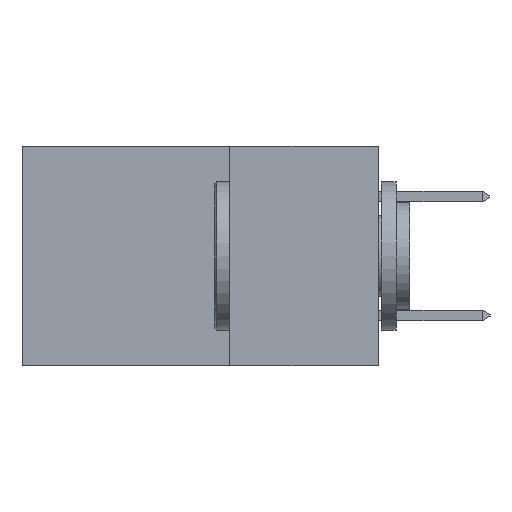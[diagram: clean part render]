
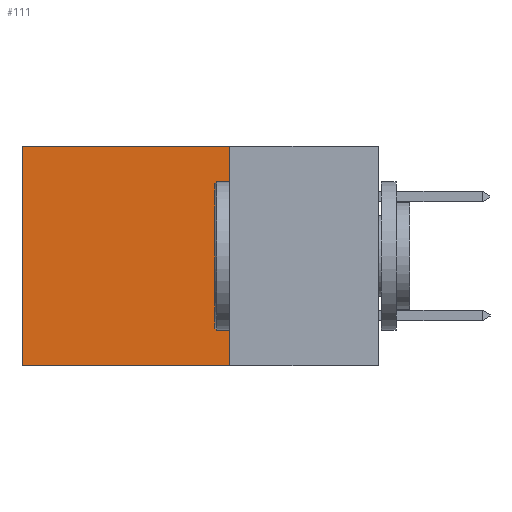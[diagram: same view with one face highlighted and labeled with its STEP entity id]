
A CAD part, left-side view. The second image highlights one B-rep face of the part: STEP entity #111.
In plain terms, the highlighted planar face has unit normal (-1, 0, 0).
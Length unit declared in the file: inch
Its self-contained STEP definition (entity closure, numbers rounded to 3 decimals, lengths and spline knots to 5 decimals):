
#111 = ADVANCED_FACE ( 'NONE', ( #12566 ), #7106, .F. ) ;
#1089 = CARTESIAN_POINT ( 'NONE',  ( 0.2615, 0.25, -0.37 ) ) ;
#1488 = EDGE_CURVE ( 'NONE', #8205, #7465, #5179, .T. ) ;
#1887 = VECTOR ( 'NONE', #9534, 39.37008 ) ;
#2770 = LINE ( 'NONE', #9122, #12770 ) ;
#3775 = CARTESIAN_POINT ( 'NONE',  ( 0.2615, 0.25, -0.37 ) ) ;
#3989 = DIRECTION ( 'NONE',  ( 0., 0., -1. ) ) ;
#4307 = EDGE_LOOP ( 'NONE', ( #10764, #14239, #8349, #5482 ) ) ;
#4802 = VERTEX_POINT ( 'NONE', #9299 ) ;
#4962 = CARTESIAN_POINT ( 'NONE',  ( 0.2615, 0.25, -0.37 ) ) ;
#5179 = LINE ( 'NONE', #13871, #1887 ) ;
#5255 = LINE ( 'NONE', #3775, #11682 ) ;
#5482 = ORIENTED_EDGE ( 'NONE', *, *, #6745, .T. ) ;
#6457 = DIRECTION ( 'NONE',  ( 0., 0., -1. ) ) ;
#6491 = DIRECTION ( 'NONE',  ( 1., 0., 0. ) ) ;
#6745 = EDGE_CURVE ( 'NONE', #4802, #8205, #14173, .T. ) ;
#7106 = PLANE ( 'NONE',  #14332 ) ;
#7465 = VERTEX_POINT ( 'NONE', #13145 ) ;
#7896 = VECTOR ( 'NONE', #8722, 39.37008 ) ;
#8205 = VERTEX_POINT ( 'NONE', #10181 ) ;
#8349 = ORIENTED_EDGE ( 'NONE', *, *, #10318, .F. ) ;
#8722 = DIRECTION ( 'NONE',  ( 0., 1., 0. ) ) ;
#8735 = DIRECTION ( 'NONE',  ( 0., 1., 0. ) ) ;
#9122 = CARTESIAN_POINT ( 'NONE',  ( 0.2615, 0.25, -0.37 ) ) ;
#9299 = CARTESIAN_POINT ( 'NONE',  ( 0.2615, 0.25, 0. ) ) ;
#9534 = DIRECTION ( 'NONE',  ( 0., 0., -1. ) ) ;
#10181 = CARTESIAN_POINT ( 'NONE',  ( 0.2615, 0.6, 0. ) ) ;
#10318 = EDGE_CURVE ( 'NONE', #4802, #11355, #5255, .T. ) ;
#10723 = EDGE_CURVE ( 'NONE', #11355, #7465, #2770, .T. ) ;
#10764 = ORIENTED_EDGE ( 'NONE', *, *, #1488, .T. ) ;
#11340 = CARTESIAN_POINT ( 'NONE',  ( 0.2615, 0.25, 0. ) ) ;
#11355 = VERTEX_POINT ( 'NONE', #1089 ) ;
#11682 = VECTOR ( 'NONE', #3989, 39.37008 ) ;
#12566 = FACE_OUTER_BOUND ( 'NONE', #4307, .T. ) ;
#12770 = VECTOR ( 'NONE', #8735, 39.37008 ) ;
#13145 = CARTESIAN_POINT ( 'NONE',  ( 0.2615, 0.6, -0.37 ) ) ;
#13871 = CARTESIAN_POINT ( 'NONE',  ( 0.2615, 0.6, -0.37 ) ) ;
#14173 = LINE ( 'NONE', #11340, #7896 ) ;
#14239 = ORIENTED_EDGE ( 'NONE', *, *, #10723, .F. ) ;
#14332 = AXIS2_PLACEMENT_3D ( 'NONE', #4962, #6491, #6457 ) ;
